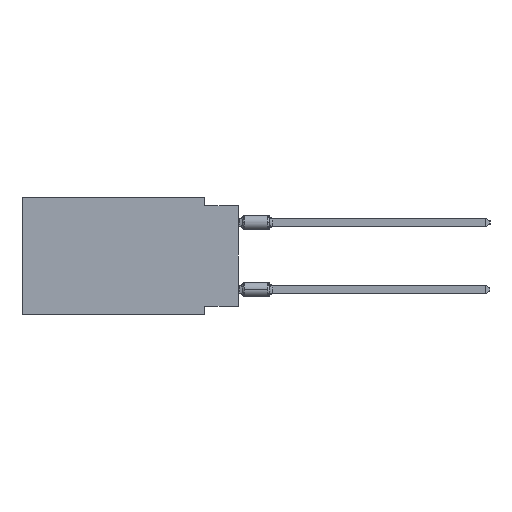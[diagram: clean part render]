
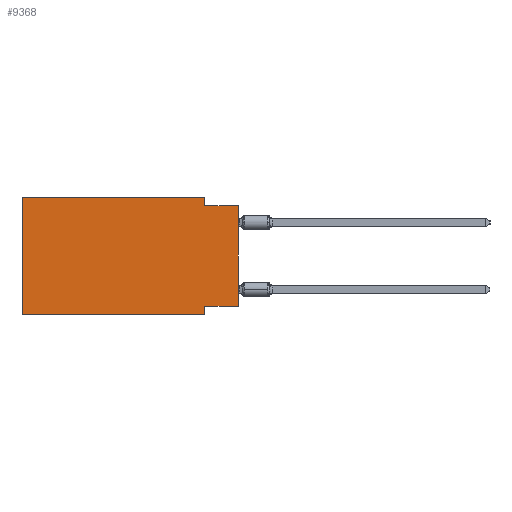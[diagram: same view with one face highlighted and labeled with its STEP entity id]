
A CAD part, left-side view. The second image highlights one B-rep face of the part: STEP entity #9368.
In plain terms, the highlighted planar face has unit normal (-1, 0, 0).
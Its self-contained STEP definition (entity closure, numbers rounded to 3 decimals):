
#105 = LINE ( 'NONE', #16831, #3401 ) ;
#327 = ORIENTED_EDGE ( 'NONE', *, *, #15375, .F. ) ;
#818 = VERTEX_POINT ( 'NONE', #23495 ) ;
#889 = EDGE_CURVE ( 'NONE', #9204, #17162, #10809, .T. ) ;
#1891 = DIRECTION ( 'NONE',  ( 0., 0., 1. ) ) ;
#2174 = EDGE_CURVE ( 'NONE', #5725, #17162, #11174, .T. ) ;
#2943 = FACE_OUTER_BOUND ( 'NONE', #14076, .T. ) ;
#3401 = VECTOR ( 'NONE', #18929, 1000. ) ;
#3425 = DIRECTION ( 'NONE',  ( 0., 0., -1. ) ) ;
#3748 = CARTESIAN_POINT ( 'NONE',  ( 0., 16.383, 0. ) ) ;
#4548 = DIRECTION ( 'NONE',  ( 0., -1., 0. ) ) ;
#4870 = DIRECTION ( 'NONE',  ( 0., 0., 1. ) ) ;
#5283 = LINE ( 'NONE', #12782, #12835 ) ;
#5725 = VERTEX_POINT ( 'NONE', #9455 ) ;
#6761 = DIRECTION ( 'NONE',  ( 1., 0., 0. ) ) ;
#7124 = CARTESIAN_POINT ( 'NONE',  ( 0., 16.383, -8.89 ) ) ;
#7429 = CARTESIAN_POINT ( 'NONE',  ( 0., 2.54, -0.635 ) ) ;
#7612 = DIRECTION ( 'NONE',  ( 0., -1., 0. ) ) ;
#8055 = VECTOR ( 'NONE', #4548, 1000. ) ;
#8211 = EDGE_CURVE ( 'NONE', #8899, #14574, #21285, .T. ) ;
#8537 = LINE ( 'NONE', #10384, #14207 ) ;
#8899 = VERTEX_POINT ( 'NONE', #3748 ) ;
#9178 = ORIENTED_EDGE ( 'NONE', *, *, #21569, .F. ) ;
#9204 = VERTEX_POINT ( 'NONE', #17105 ) ;
#9368 = ADVANCED_FACE ( 'NONE', ( #2943 ), #23137, .F. ) ;
#9455 = CARTESIAN_POINT ( 'NONE',  ( 0., 2.54, -8.255 ) ) ;
#9601 = ORIENTED_EDGE ( 'NONE', *, *, #16775, .T. ) ;
#9621 = VERTEX_POINT ( 'NONE', #13260 ) ;
#9626 = ORIENTED_EDGE ( 'NONE', *, *, #889, .T. ) ;
#10354 = CARTESIAN_POINT ( 'NONE',  ( 0., 2.54, 0. ) ) ;
#10384 = CARTESIAN_POINT ( 'NONE',  ( 0., 0., -0.635 ) ) ;
#10809 = LINE ( 'NONE', #7124, #13804 ) ;
#11174 = LINE ( 'NONE', #20894, #22110 ) ;
#11526 = VERTEX_POINT ( 'NONE', #7429 ) ;
#12669 = ORIENTED_EDGE ( 'NONE', *, *, #23478, .F. ) ;
#12782 = CARTESIAN_POINT ( 'NONE',  ( 0., 2.54, 0. ) ) ;
#12835 = VECTOR ( 'NONE', #3425, 1000. ) ;
#12963 = CARTESIAN_POINT ( 'NONE',  ( 0., 16.383, 0. ) ) ;
#13260 = CARTESIAN_POINT ( 'NONE',  ( 0., 0., -0.635 ) ) ;
#13387 = DIRECTION ( 'NONE',  ( 0., 0., -1. ) ) ;
#13804 = VECTOR ( 'NONE', #7612, 1000. ) ;
#14026 = CARTESIAN_POINT ( 'NONE',  ( 0., 16.383, 0. ) ) ;
#14076 = EDGE_LOOP ( 'NONE', ( #9601, #327, #16160, #20329, #12669, #9626, #18756, #9178 ) ) ;
#14207 = VECTOR ( 'NONE', #19852, 1000. ) ;
#14266 = DIRECTION ( 'NONE',  ( 0., 0., -1. ) ) ;
#14574 = VERTEX_POINT ( 'NONE', #10354 ) ;
#15375 = EDGE_CURVE ( 'NONE', #11526, #9621, #8537, .T. ) ;
#16160 = ORIENTED_EDGE ( 'NONE', *, *, #21457, .F. ) ;
#16775 = EDGE_CURVE ( 'NONE', #818, #9621, #21609, .T. ) ;
#16831 = CARTESIAN_POINT ( 'NONE',  ( 0., 0., -8.255 ) ) ;
#17105 = CARTESIAN_POINT ( 'NONE',  ( 0., 16.383, -8.89 ) ) ;
#17162 = VERTEX_POINT ( 'NONE', #17857 ) ;
#17586 = CARTESIAN_POINT ( 'NONE',  ( 0., 16.383, 0. ) ) ;
#17857 = CARTESIAN_POINT ( 'NONE',  ( 0., 2.54, -8.89 ) ) ;
#18748 = VECTOR ( 'NONE', #1891, 1000. ) ;
#18756 = ORIENTED_EDGE ( 'NONE', *, *, #2174, .F. ) ;
#18929 = DIRECTION ( 'NONE',  ( 0., 1., 0. ) ) ;
#19852 = DIRECTION ( 'NONE',  ( 0., -1., 0. ) ) ;
#20329 = ORIENTED_EDGE ( 'NONE', *, *, #8211, .F. ) ;
#20717 = LINE ( 'NONE', #12963, #18748 ) ;
#20894 = CARTESIAN_POINT ( 'NONE',  ( 0., 2.54, -8.89 ) ) ;
#21255 = VECTOR ( 'NONE', #4870, 1000. ) ;
#21285 = LINE ( 'NONE', #17586, #8055 ) ;
#21457 = EDGE_CURVE ( 'NONE', #14574, #11526, #5283, .T. ) ;
#21569 = EDGE_CURVE ( 'NONE', #818, #5725, #105, .T. ) ;
#21609 = LINE ( 'NONE', #23335, #21255 ) ;
#22110 = VECTOR ( 'NONE', #13387, 1000. ) ;
#23137 = PLANE ( 'NONE',  #24209 ) ;
#23335 = CARTESIAN_POINT ( 'NONE',  ( 0., 0., 0. ) ) ;
#23478 = EDGE_CURVE ( 'NONE', #9204, #8899, #20717, .T. ) ;
#23495 = CARTESIAN_POINT ( 'NONE',  ( 0., 0., -8.255 ) ) ;
#24209 = AXIS2_PLACEMENT_3D ( 'NONE', #14026, #6761, #14266 ) ;
